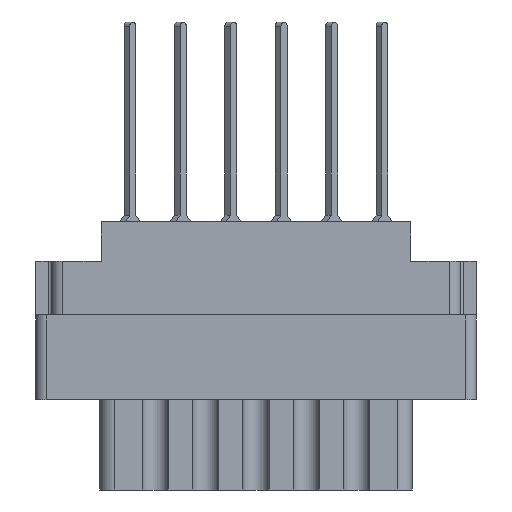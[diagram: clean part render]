
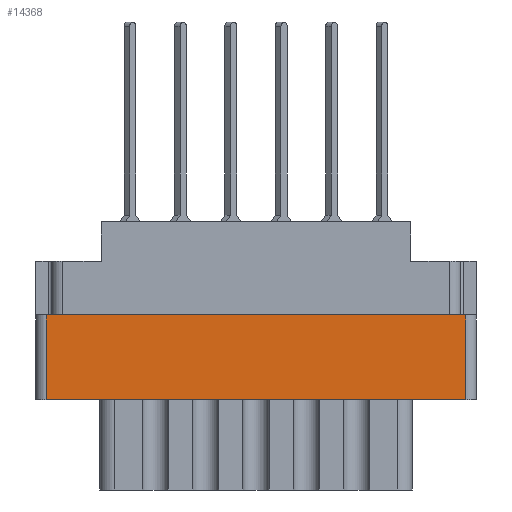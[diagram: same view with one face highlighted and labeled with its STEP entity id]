
A CAD part, front view. The second image highlights one B-rep face of the part: STEP entity #14368.
In plain terms, the highlighted planar face has unit normal (0, -1, 0).
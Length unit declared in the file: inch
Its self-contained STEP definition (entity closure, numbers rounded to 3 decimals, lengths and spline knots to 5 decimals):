
#461 = LINE ( 'NONE', #12267, #19002 ) ;
#1040 = CARTESIAN_POINT ( 'NONE',  ( -0.624, -0.343, -0.529 ) ) ;
#1130 = VERTEX_POINT ( 'NONE', #1040 ) ;
#1274 = ORIENTED_EDGE ( 'NONE', *, *, #4997, .F. ) ;
#2001 = VERTEX_POINT ( 'NONE', #5271 ) ;
#2279 = VERTEX_POINT ( 'NONE', #17777 ) ;
#3066 = DIRECTION ( 'NONE',  ( 0., 0., 1. ) ) ;
#3633 = ORIENTED_EDGE ( 'NONE', *, *, #16613, .F. ) ;
#3688 = VECTOR ( 'NONE', #3066, 39.37008 ) ;
#3805 = DIRECTION ( 'NONE',  ( 1., 0., 0. ) ) ;
#4095 = CARTESIAN_POINT ( 'NONE',  ( -0.656, -0.343, -0.277 ) ) ;
#4805 = CARTESIAN_POINT ( 'NONE',  ( -0.624, -0.343, -0.798 ) ) ;
#4997 = EDGE_CURVE ( 'NONE', #18198, #1130, #461, .T. ) ;
#5271 = CARTESIAN_POINT ( 'NONE',  ( 0.624, -0.343, -0.277 ) ) ;
#5537 = PLANE ( 'NONE',  #17744 ) ;
#5818 = CARTESIAN_POINT ( 'NONE',  ( -0.624, -0.343, -0.798 ) ) ;
#7420 = DIRECTION ( 'NONE',  ( 0., 0., 1. ) ) ;
#8303 = EDGE_CURVE ( 'NONE', #18198, #2001, #15088, .T. ) ;
#8736 = FACE_OUTER_BOUND ( 'NONE', #18157, .T. ) ;
#8830 = DIRECTION ( 'NONE',  ( 0., 0., -1. ) ) ;
#9029 = VECTOR ( 'NONE', #3805, 39.37008 ) ;
#9126 = ORIENTED_EDGE ( 'NONE', *, *, #11190, .F. ) ;
#9258 = CARTESIAN_POINT ( 'NONE',  ( 0.624, -0.343, -0.798 ) ) ;
#9994 = ORIENTED_EDGE ( 'NONE', *, *, #8303, .T. ) ;
#10159 = VECTOR ( 'NONE', #7420, 39.37008 ) ;
#10712 = LINE ( 'NONE', #4805, #10159 ) ;
#11190 = EDGE_CURVE ( 'NONE', #2279, #2001, #15924, .T. ) ;
#12267 = CARTESIAN_POINT ( 'NONE',  ( 0.624, -0.343, -0.529 ) ) ;
#14368 = ADVANCED_FACE ( 'NONE', ( #8736 ), #5537, .T. ) ;
#15088 = LINE ( 'NONE', #9258, #3688 ) ;
#15924 = LINE ( 'NONE', #4095, #9029 ) ;
#16613 = EDGE_CURVE ( 'NONE', #1130, #2279, #10712, .T. ) ;
#17174 = CARTESIAN_POINT ( 'NONE',  ( 0.624, -0.343, -0.529 ) ) ;
#17469 = DIRECTION ( 'NONE',  ( 0., -1., 0. ) ) ;
#17744 = AXIS2_PLACEMENT_3D ( 'NONE', #5818, #17469, #8830 ) ;
#17777 = CARTESIAN_POINT ( 'NONE',  ( -0.624, -0.343, -0.277 ) ) ;
#18157 = EDGE_LOOP ( 'NONE', ( #3633, #1274, #9994, #9126 ) ) ;
#18179 = DIRECTION ( 'NONE',  ( -1., 0., 0. ) ) ;
#18198 = VERTEX_POINT ( 'NONE', #17174 ) ;
#19002 = VECTOR ( 'NONE', #18179, 39.37008 ) ;
